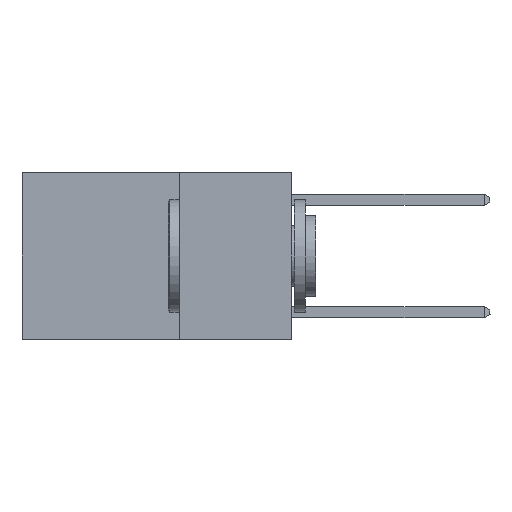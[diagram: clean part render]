
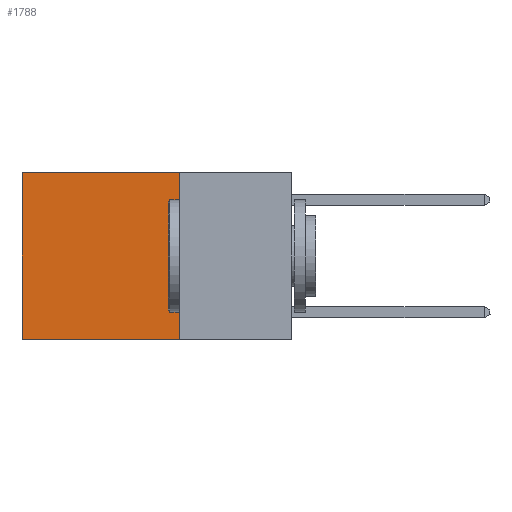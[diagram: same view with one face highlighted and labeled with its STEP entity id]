
A CAD part, left-side view. The second image highlights one B-rep face of the part: STEP entity #1788.
In plain terms, the highlighted planar face has unit normal (-1, 0, 0).
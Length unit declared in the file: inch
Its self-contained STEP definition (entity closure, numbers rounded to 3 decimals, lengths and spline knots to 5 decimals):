
#112 = DIRECTION ( 'NONE',  ( 0., 0., -1. ) ) ;
#229 = EDGE_LOOP ( 'NONE', ( #968, #11481, #8505, #6231 ) ) ;
#348 = VERTEX_POINT ( 'NONE', #7217 ) ;
#420 = VECTOR ( 'NONE', #6502, 39.37008 ) ;
#754 = LINE ( 'NONE', #1401, #420 ) ;
#899 = EDGE_CURVE ( 'NONE', #348, #2280, #9901, .T. ) ;
#968 = ORIENTED_EDGE ( 'NONE', *, *, #4775, .T. ) ;
#1401 = CARTESIAN_POINT ( 'NONE',  ( 0.2625, 0.25, 0. ) ) ;
#1788 = ADVANCED_FACE ( 'NONE', ( #7227 ), #13006, .F. ) ;
#1932 = CARTESIAN_POINT ( 'NONE',  ( 0.2625, 0.25, 0. ) ) ;
#2280 = VERTEX_POINT ( 'NONE', #5968 ) ;
#3574 = DIRECTION ( 'NONE',  ( 1., 0., 0. ) ) ;
#3791 = VERTEX_POINT ( 'NONE', #3796 ) ;
#3796 = CARTESIAN_POINT ( 'NONE',  ( 0.2625, 0.6, 0. ) ) ;
#3814 = EDGE_CURVE ( 'NONE', #5640, #3791, #8147, .T. ) ;
#4702 = CARTESIAN_POINT ( 'NONE',  ( 0.2625, 0.25, 0. ) ) ;
#4757 = EDGE_CURVE ( 'NONE', #5640, #348, #754, .T. ) ;
#4775 = EDGE_CURVE ( 'NONE', #3791, #2280, #8641, .T. ) ;
#5424 = VECTOR ( 'NONE', #9970, 39.37008 ) ;
#5640 = VERTEX_POINT ( 'NONE', #4702 ) ;
#5686 = AXIS2_PLACEMENT_3D ( 'NONE', #1932, #3574, #112 ) ;
#5850 = CARTESIAN_POINT ( 'NONE',  ( 0.2625, 0.25, 0. ) ) ;
#5968 = CARTESIAN_POINT ( 'NONE',  ( 0.2625, 0.6, -0.37 ) ) ;
#6231 = ORIENTED_EDGE ( 'NONE', *, *, #3814, .T. ) ;
#6502 = DIRECTION ( 'NONE',  ( 0., 0., -1. ) ) ;
#7217 = CARTESIAN_POINT ( 'NONE',  ( 0.2625, 0.25, -0.37 ) ) ;
#7227 = FACE_OUTER_BOUND ( 'NONE', #229, .T. ) ;
#8147 = LINE ( 'NONE', #5850, #5424 ) ;
#8313 = VECTOR ( 'NONE', #11595, 39.37008 ) ;
#8505 = ORIENTED_EDGE ( 'NONE', *, *, #4757, .F. ) ;
#8641 = LINE ( 'NONE', #12550, #8313 ) ;
#9901 = LINE ( 'NONE', #10603, #12496 ) ;
#9937 = DIRECTION ( 'NONE',  ( 0., 1., 0. ) ) ;
#9970 = DIRECTION ( 'NONE',  ( 0., 1., 0. ) ) ;
#10603 = CARTESIAN_POINT ( 'NONE',  ( 0.2625, 0.25, -0.37 ) ) ;
#11481 = ORIENTED_EDGE ( 'NONE', *, *, #899, .F. ) ;
#11595 = DIRECTION ( 'NONE',  ( 0., 0., -1. ) ) ;
#12496 = VECTOR ( 'NONE', #9937, 39.37008 ) ;
#12550 = CARTESIAN_POINT ( 'NONE',  ( 0.2625, 0.6, 0. ) ) ;
#13006 = PLANE ( 'NONE',  #5686 ) ;
